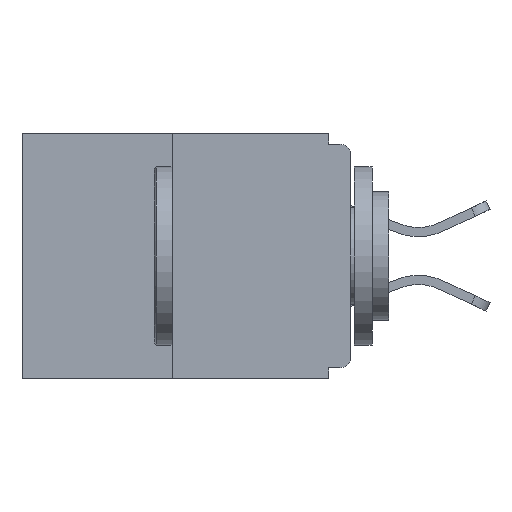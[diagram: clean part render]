
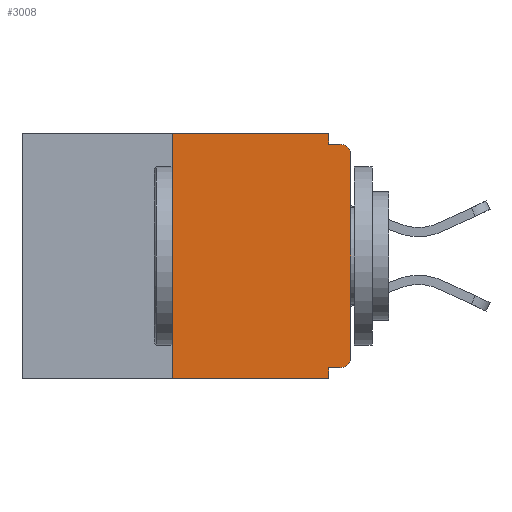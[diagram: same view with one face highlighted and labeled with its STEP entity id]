
A CAD part, left-side view. The second image highlights one B-rep face of the part: STEP entity #3008.
In plain terms, the highlighted planar face has unit normal (-1, 0, 0).
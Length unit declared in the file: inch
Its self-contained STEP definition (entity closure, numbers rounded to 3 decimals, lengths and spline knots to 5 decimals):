
#45 = LINE ( 'NONE', #19527, #18501 ) ;
#98 = DIRECTION ( 'NONE',  ( 0., 1., 0. ) ) ;
#364 = VERTEX_POINT ( 'NONE', #19818 ) ;
#788 = EDGE_CURVE ( 'NONE', #12507, #18783, #5255, .T. ) ;
#967 = DIRECTION ( 'NONE',  ( 1., 0., 0. ) ) ;
#1010 = CARTESIAN_POINT ( 'NONE',  ( 0., 0.031, -0.015 ) ) ;
#1032 = PLANE ( 'NONE',  #13114 ) ;
#1275 = CARTESIAN_POINT ( 'NONE',  ( 0., 0.031, 0. ) ) ;
#1751 = DIRECTION ( 'NONE',  ( -1., 0., 0. ) ) ;
#1879 = VECTOR ( 'NONE', #7163, 39.37008 ) ;
#1952 = CARTESIAN_POINT ( 'NONE',  ( 0., 0.015, -0.328 ) ) ;
#2430 = EDGE_CURVE ( 'NONE', #12944, #15876, #7994, .T. ) ;
#2796 = LINE ( 'NONE', #18791, #16439 ) ;
#2823 = CIRCLE ( 'NONE', #15879, 0.015 ) ;
#3008 = ADVANCED_FACE ( 'NONE', ( #3017 ), #1032, .F. ) ;
#3017 = FACE_OUTER_BOUND ( 'NONE', #16368, .T. ) ;
#3259 = DIRECTION ( 'NONE',  ( 0., 0., 1. ) ) ;
#3319 = DIRECTION ( 'NONE',  ( 0., 0., -1. ) ) ;
#3679 = CARTESIAN_POINT ( 'NONE',  ( 0., 0.031, -0.343 ) ) ;
#3850 = DIRECTION ( 'NONE',  ( 0., 0., -1. ) ) ;
#4105 = ORIENTED_EDGE ( 'NONE', *, *, #2430, .F. ) ;
#4208 = CARTESIAN_POINT ( 'NONE',  ( 0., 0.031, -0.343 ) ) ;
#4272 = ORIENTED_EDGE ( 'NONE', *, *, #788, .F. ) ;
#4357 = LINE ( 'NONE', #12275, #12233 ) ;
#4736 = LINE ( 'NONE', #4208, #11914 ) ;
#5174 = ORIENTED_EDGE ( 'NONE', *, *, #17269, .T. ) ;
#5255 = LINE ( 'NONE', #18780, #17200 ) ;
#5297 = DIRECTION ( 'NONE',  ( -1., 0., 0. ) ) ;
#5410 = EDGE_CURVE ( 'NONE', #6715, #364, #4357, .T. ) ;
#5818 = CARTESIAN_POINT ( 'NONE',  ( 0., 0.25, 0. ) ) ;
#5912 = VERTEX_POINT ( 'NONE', #3679 ) ;
#6625 = ORIENTED_EDGE ( 'NONE', *, *, #8109, .T. ) ;
#6670 = ORIENTED_EDGE ( 'NONE', *, *, #10626, .T. ) ;
#6715 = VERTEX_POINT ( 'NONE', #7150 ) ;
#6749 = CARTESIAN_POINT ( 'NONE',  ( 0., 0.031, -0.328 ) ) ;
#7150 = CARTESIAN_POINT ( 'NONE',  ( 0., 0., -0.313 ) ) ;
#7163 = DIRECTION ( 'NONE',  ( 0., -1., 0. ) ) ;
#7503 = CARTESIAN_POINT ( 'NONE',  ( 0., 0.015, -0.015 ) ) ;
#7994 = LINE ( 'NONE', #8330, #10404 ) ;
#8109 = EDGE_CURVE ( 'NONE', #12507, #6715, #2823, .T. ) ;
#8167 = CIRCLE ( 'NONE', #17948, 0.015 ) ;
#8330 = CARTESIAN_POINT ( 'NONE',  ( 0., 0.031, 0. ) ) ;
#9613 = DIRECTION ( 'NONE',  ( 0., -1., 0. ) ) ;
#9996 = LINE ( 'NONE', #14822, #1879 ) ;
#10010 = CARTESIAN_POINT ( 'NONE',  ( 0., 0.46, 0. ) ) ;
#10404 = VECTOR ( 'NONE', #3850, 39.37008 ) ;
#10626 = EDGE_CURVE ( 'NONE', #364, #11804, #8167, .T. ) ;
#10659 = ORIENTED_EDGE ( 'NONE', *, *, #15225, .F. ) ;
#11081 = VECTOR ( 'NONE', #13060, 39.37008 ) ;
#11804 = VERTEX_POINT ( 'NONE', #7503 ) ;
#11803 = DIRECTION ( 'NONE',  ( 0., -1., 0. ) ) ;
#11914 = VECTOR ( 'NONE', #14907, 39.37008 ) ;
#12233 = VECTOR ( 'NONE', #3259, 39.37008 ) ;
#12275 = CARTESIAN_POINT ( 'NONE',  ( 0., 0., 0. ) ) ;
#12507 = VERTEX_POINT ( 'NONE', #1952 ) ;
#12675 = VERTEX_POINT ( 'NONE', #5818 ) ;
#12944 = VERTEX_POINT ( 'NONE', #1275 ) ;
#12978 = EDGE_CURVE ( 'NONE', #18783, #5912, #4736, .T. ) ;
#12987 = CARTESIAN_POINT ( 'NONE',  ( 0., 0.25, -0.343 ) ) ;
#13060 = DIRECTION ( 'NONE',  ( 0., 0., 1. ) ) ;
#13114 = AXIS2_PLACEMENT_3D ( 'NONE', #10010, #967, #14935 ) ;
#14033 = ORIENTED_EDGE ( 'NONE', *, *, #16015, .F. ) ;
#14202 = EDGE_CURVE ( 'NONE', #12675, #12944, #2796, .T. ) ;
#14268 = VERTEX_POINT ( 'NONE', #12987 ) ;
#14390 = CARTESIAN_POINT ( 'NONE',  ( 0., 0.25, 0. ) ) ;
#14822 = CARTESIAN_POINT ( 'NONE',  ( 0., 0.46, -0.343 ) ) ;
#14907 = DIRECTION ( 'NONE',  ( 0., 0., -1. ) ) ;
#14935 = DIRECTION ( 'NONE',  ( 0., 0., -1. ) ) ;
#15225 = EDGE_CURVE ( 'NONE', #14268, #12675, #19274, .T. ) ;
#15691 = CARTESIAN_POINT ( 'NONE',  ( 0., 0.015, -0.313 ) ) ;
#15876 = VERTEX_POINT ( 'NONE', #1010 ) ;
#15879 = AXIS2_PLACEMENT_3D ( 'NONE', #15691, #1751, #3319 ) ;
#16015 = EDGE_CURVE ( 'NONE', #15876, #11804, #45, .T. ) ;
#16368 = EDGE_LOOP ( 'NONE', ( #19521, #10659, #5174, #17843, #4272, #6625, #16576, #6670, #14033, #4105 ) ) ;
#16439 = VECTOR ( 'NONE', #9613, 39.37008 ) ;
#16576 = ORIENTED_EDGE ( 'NONE', *, *, #5410, .T. ) ;
#17200 = VECTOR ( 'NONE', #98, 39.37008 ) ;
#17269 = EDGE_CURVE ( 'NONE', #14268, #5912, #9996, .T. ) ;
#17310 = CARTESIAN_POINT ( 'NONE',  ( 0., 0.015, -0.03 ) ) ;
#17518 = DIRECTION ( 'NONE',  ( 0., 0., -1. ) ) ;
#17843 = ORIENTED_EDGE ( 'NONE', *, *, #12978, .F. ) ;
#17948 = AXIS2_PLACEMENT_3D ( 'NONE', #17310, #5297, #17518 ) ;
#18501 = VECTOR ( 'NONE', #11803, 39.37008 ) ;
#18780 = CARTESIAN_POINT ( 'NONE',  ( 0., 0., -0.328 ) ) ;
#18783 = VERTEX_POINT ( 'NONE', #6749 ) ;
#18791 = CARTESIAN_POINT ( 'NONE',  ( 0., 0.46, 0. ) ) ;
#19274 = LINE ( 'NONE', #14390, #11081 ) ;
#19521 = ORIENTED_EDGE ( 'NONE', *, *, #14202, .F. ) ;
#19527 = CARTESIAN_POINT ( 'NONE',  ( 0., 0., -0.015 ) ) ;
#19818 = CARTESIAN_POINT ( 'NONE',  ( 0., 0., -0.03 ) ) ;
